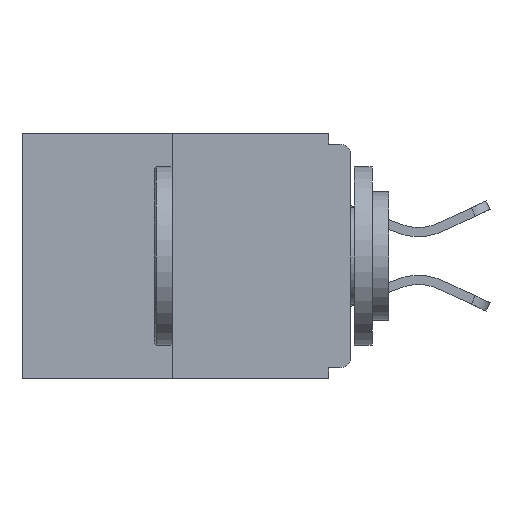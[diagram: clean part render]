
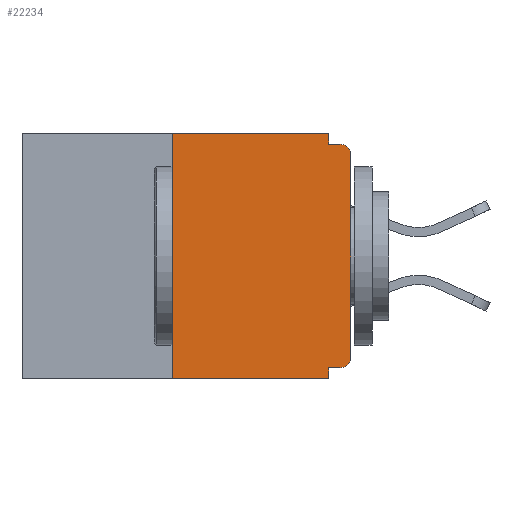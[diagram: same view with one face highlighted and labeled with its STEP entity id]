
A CAD part, left-side view. The second image highlights one B-rep face of the part: STEP entity #22234.
In plain terms, the highlighted planar face has unit normal (-1, 0, 0).
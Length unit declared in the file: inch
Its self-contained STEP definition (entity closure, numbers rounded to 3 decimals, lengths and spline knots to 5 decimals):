
#518 = DIRECTION ( 'NONE',  ( -1., 0., 0. ) ) ;
#1010 = EDGE_CURVE ( 'NONE', #21587, #2534, #10911, .T. ) ;
#1193 = VECTOR ( 'NONE', #3140, 39.37008 ) ;
#1284 = VECTOR ( 'NONE', #14829, 39.37008 ) ;
#1526 = CIRCLE ( 'NONE', #10014, 0.015 ) ;
#2050 = VECTOR ( 'NONE', #13228, 39.37008 ) ;
#2248 = ORIENTED_EDGE ( 'NONE', *, *, #7136, .F. ) ;
#2268 = EDGE_CURVE ( 'NONE', #14956, #12305, #4016, .T. ) ;
#2388 = EDGE_CURVE ( 'NONE', #16649, #16429, #7576, .T. ) ;
#2436 = EDGE_CURVE ( 'NONE', #20150, #21587, #9024, .T. ) ;
#2478 = ORIENTED_EDGE ( 'NONE', *, *, #2268, .F. ) ;
#2489 = CARTESIAN_POINT ( 'NONE',  ( 0., 0.015, -0.313 ) ) ;
#2534 = VERTEX_POINT ( 'NONE', #23563 ) ;
#2733 = DIRECTION ( 'NONE',  ( 0., 0., 1. ) ) ;
#3140 = DIRECTION ( 'NONE',  ( 0., 0., -1. ) ) ;
#3295 = CARTESIAN_POINT ( 'NONE',  ( 0., 0., -0.03 ) ) ;
#3618 = LINE ( 'NONE', #5436, #12513 ) ;
#4016 = LINE ( 'NONE', #11204, #23998 ) ;
#4700 = CARTESIAN_POINT ( 'NONE',  ( 0., 0.25, 0. ) ) ;
#5122 = DIRECTION ( 'NONE',  ( -1., 0., 0. ) ) ;
#5209 = FACE_OUTER_BOUND ( 'NONE', #8589, .T. ) ;
#5266 = EDGE_CURVE ( 'NONE', #7150, #2534, #18524, .T. ) ;
#5436 = CARTESIAN_POINT ( 'NONE',  ( 0., 0.46, 0. ) ) ;
#5574 = CARTESIAN_POINT ( 'NONE',  ( 0., 0.46, -0.343 ) ) ;
#5987 = CARTESIAN_POINT ( 'NONE',  ( 0., 0., -0.328 ) ) ;
#6383 = VECTOR ( 'NONE', #8039, 39.37008 ) ;
#6788 = CARTESIAN_POINT ( 'NONE',  ( 0., 0.031, 0. ) ) ;
#7136 = EDGE_CURVE ( 'NONE', #20406, #14956, #16061, .T. ) ;
#7150 = VERTEX_POINT ( 'NONE', #12447 ) ;
#7576 = LINE ( 'NONE', #19318, #18310 ) ;
#7881 = DIRECTION ( 'NONE',  ( 0., 0., 1. ) ) ;
#7948 = ORIENTED_EDGE ( 'NONE', *, *, #2388, .T. ) ;
#8008 = CARTESIAN_POINT ( 'NONE',  ( 0., 0.25, 0. ) ) ;
#8014 = CARTESIAN_POINT ( 'NONE',  ( 0., 0.015, -0.015 ) ) ;
#8035 = DIRECTION ( 'NONE',  ( 0., 0., -1. ) ) ;
#8039 = DIRECTION ( 'NONE',  ( 0., 1., 0. ) ) ;
#8333 = AXIS2_PLACEMENT_3D ( 'NONE', #11254, #22720, #9090 ) ;
#8442 = CARTESIAN_POINT ( 'NONE',  ( 0., 0., -0.313 ) ) ;
#8589 = EDGE_LOOP ( 'NONE', ( #17829, #15133, #9141, #23463, #16107, #19085, #7948, #14707, #2478, #2248 ) ) ;
#9024 = LINE ( 'NONE', #5987, #6383 ) ;
#9090 = DIRECTION ( 'NONE',  ( 0., 0., -1. ) ) ;
#9141 = ORIENTED_EDGE ( 'NONE', *, *, #5266, .T. ) ;
#9454 = CARTESIAN_POINT ( 'NONE',  ( 0., 0.031, -0.015 ) ) ;
#10012 = CARTESIAN_POINT ( 'NONE',  ( 0., 0.015, -0.328 ) ) ;
#10014 = AXIS2_PLACEMENT_3D ( 'NONE', #20120, #5122, #10489 ) ;
#10489 = DIRECTION ( 'NONE',  ( 0., 0., -1. ) ) ;
#10911 = LINE ( 'NONE', #24607, #2050 ) ;
#11056 = VERTEX_POINT ( 'NONE', #8008 ) ;
#11204 = CARTESIAN_POINT ( 'NONE',  ( 0., 0., -0.015 ) ) ;
#11254 = CARTESIAN_POINT ( 'NONE',  ( 0., 0.46, 0. ) ) ;
#12305 = VERTEX_POINT ( 'NONE', #8014 ) ;
#12447 = CARTESIAN_POINT ( 'NONE',  ( 0., 0.25, -0.343 ) ) ;
#12513 = VECTOR ( 'NONE', #22688, 39.37008 ) ;
#13228 = DIRECTION ( 'NONE',  ( 0., 0., -1. ) ) ;
#14415 = AXIS2_PLACEMENT_3D ( 'NONE', #2489, #518, #8035 ) ;
#14707 = ORIENTED_EDGE ( 'NONE', *, *, #19589, .T. ) ;
#14829 = DIRECTION ( 'NONE',  ( 0., -1., 0. ) ) ;
#14956 = VERTEX_POINT ( 'NONE', #9454 ) ;
#15133 = ORIENTED_EDGE ( 'NONE', *, *, #24051, .F. ) ;
#15962 = EDGE_CURVE ( 'NONE', #11056, #20406, #3618, .T. ) ;
#16061 = LINE ( 'NONE', #6788, #1193 ) ;
#16107 = ORIENTED_EDGE ( 'NONE', *, *, #2436, .F. ) ;
#16429 = VERTEX_POINT ( 'NONE', #3295 ) ;
#16649 = VERTEX_POINT ( 'NONE', #8442 ) ;
#17829 = ORIENTED_EDGE ( 'NONE', *, *, #15962, .F. ) ;
#18310 = VECTOR ( 'NONE', #7881, 39.37008 ) ;
#18524 = LINE ( 'NONE', #5574, #1284 ) ;
#19085 = ORIENTED_EDGE ( 'NONE', *, *, #23830, .T. ) ;
#19318 = CARTESIAN_POINT ( 'NONE',  ( 0., 0., 0. ) ) ;
#19589 = EDGE_CURVE ( 'NONE', #16429, #12305, #1526, .T. ) ;
#19707 = VECTOR ( 'NONE', #2733, 39.37008 ) ;
#20120 = CARTESIAN_POINT ( 'NONE',  ( 0., 0.015, -0.03 ) ) ;
#20150 = VERTEX_POINT ( 'NONE', #10012 ) ;
#20406 = VERTEX_POINT ( 'NONE', #22987 ) ;
#20725 = PLANE ( 'NONE',  #8333 ) ;
#20753 = DIRECTION ( 'NONE',  ( 0., -1., 0. ) ) ;
#20836 = CARTESIAN_POINT ( 'NONE',  ( 0., 0.031, -0.328 ) ) ;
#21587 = VERTEX_POINT ( 'NONE', #20836 ) ;
#22234 = ADVANCED_FACE ( 'NONE', ( #5209 ), #20725, .F. ) ;
#22688 = DIRECTION ( 'NONE',  ( 0., -1., 0. ) ) ;
#22720 = DIRECTION ( 'NONE',  ( 1., 0., 0. ) ) ;
#22987 = CARTESIAN_POINT ( 'NONE',  ( 0., 0.031, 0. ) ) ;
#23000 = LINE ( 'NONE', #4700, #19707 ) ;
#23463 = ORIENTED_EDGE ( 'NONE', *, *, #1010, .F. ) ;
#23563 = CARTESIAN_POINT ( 'NONE',  ( 0., 0.031, -0.343 ) ) ;
#23830 = EDGE_CURVE ( 'NONE', #20150, #16649, #24221, .T. ) ;
#23998 = VECTOR ( 'NONE', #20753, 39.37008 ) ;
#24051 = EDGE_CURVE ( 'NONE', #7150, #11056, #23000, .T. ) ;
#24221 = CIRCLE ( 'NONE', #14415, 0.015 ) ;
#24607 = CARTESIAN_POINT ( 'NONE',  ( 0., 0.031, -0.343 ) ) ;
